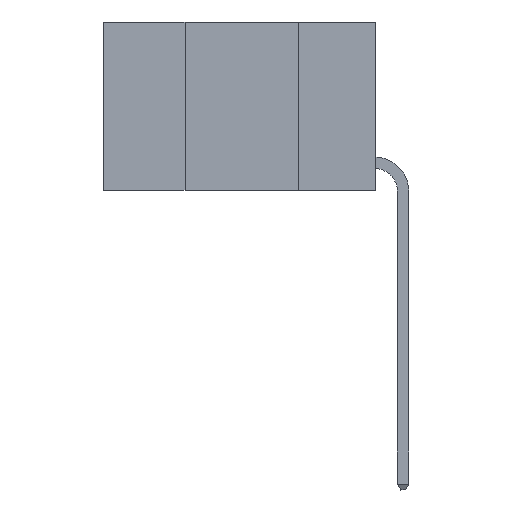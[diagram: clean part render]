
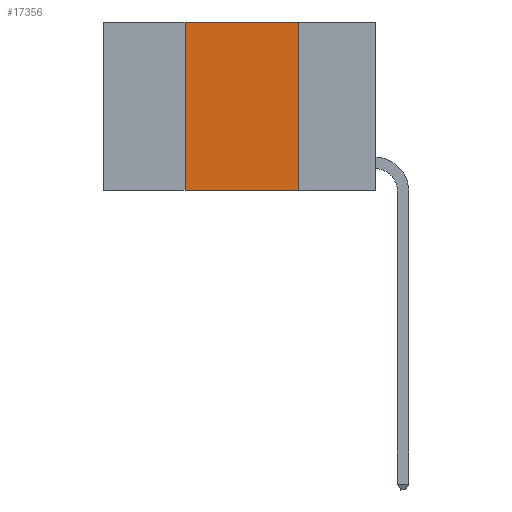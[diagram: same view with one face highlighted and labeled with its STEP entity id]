
A CAD part, left-side view. The second image highlights one B-rep face of the part: STEP entity #17356.
In plain terms, the highlighted planar face has unit normal (-1, 0, 0).
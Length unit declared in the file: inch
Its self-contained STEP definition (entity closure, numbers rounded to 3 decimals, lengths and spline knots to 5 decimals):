
#226 = EDGE_CURVE ( 'NONE', #10276, #16481, #4317, .T. ) ;
#534 = VECTOR ( 'NONE', #7224, 39.37008 ) ;
#743 = DIRECTION ( 'NONE',  ( 1., 0., 0. ) ) ;
#1006 = CARTESIAN_POINT ( 'NONE',  ( 0., 0.6, 0. ) ) ;
#1382 = CARTESIAN_POINT ( 'NONE',  ( 0., 0.42, -0.37 ) ) ;
#2932 = VECTOR ( 'NONE', #10720, 39.37008 ) ;
#3432 = CARTESIAN_POINT ( 'NONE',  ( 0., 0.42, 0. ) ) ;
#4302 = CARTESIAN_POINT ( 'NONE',  ( 0., 0.6, 0. ) ) ;
#4309 = EDGE_LOOP ( 'NONE', ( #8453, #10010, #6700, #13019 ) ) ;
#4317 = LINE ( 'NONE', #16636, #534 ) ;
#4450 = LINE ( 'NONE', #5895, #8663 ) ;
#4483 = EDGE_CURVE ( 'NONE', #10280, #13023, #10051, .T. ) ;
#4573 = CARTESIAN_POINT ( 'NONE',  ( 0., 0.17, 0. ) ) ;
#4577 = DIRECTION ( 'NONE',  ( 0., -1., 0. ) ) ;
#5895 = CARTESIAN_POINT ( 'NONE',  ( 0., 0.17, 0. ) ) ;
#6700 = ORIENTED_EDGE ( 'NONE', *, *, #14070, .F. ) ;
#6731 = EDGE_CURVE ( 'NONE', #13023, #16481, #4450, .T. ) ;
#7224 = DIRECTION ( 'NONE',  ( 0., -1., 0. ) ) ;
#8453 = ORIENTED_EDGE ( 'NONE', *, *, #6731, .F. ) ;
#8663 = VECTOR ( 'NONE', #17027, 39.37008 ) ;
#8890 = AXIS2_PLACEMENT_3D ( 'NONE', #1006, #743, #9052 ) ;
#9052 = DIRECTION ( 'NONE',  ( 0., 0., -1. ) ) ;
#9147 = FACE_OUTER_BOUND ( 'NONE', #4309, .T. ) ;
#9238 = PLANE ( 'NONE',  #8890 ) ;
#10010 = ORIENTED_EDGE ( 'NONE', *, *, #4483, .F. ) ;
#10051 = LINE ( 'NONE', #4302, #12652 ) ;
#10276 = VERTEX_POINT ( 'NONE', #1382 ) ;
#10280 = VERTEX_POINT ( 'NONE', #16709 ) ;
#10720 = DIRECTION ( 'NONE',  ( 0., 0., 1. ) ) ;
#12652 = VECTOR ( 'NONE', #4577, 39.37008 ) ;
#13019 = ORIENTED_EDGE ( 'NONE', *, *, #226, .T. ) ;
#13023 = VERTEX_POINT ( 'NONE', #4573 ) ;
#13901 = CARTESIAN_POINT ( 'NONE',  ( 0., 0.17, -0.37 ) ) ;
#14070 = EDGE_CURVE ( 'NONE', #10276, #10280, #14819, .T. ) ;
#14819 = LINE ( 'NONE', #3432, #2932 ) ;
#16481 = VERTEX_POINT ( 'NONE', #13901 ) ;
#16636 = CARTESIAN_POINT ( 'NONE',  ( 0., 0.6, -0.37 ) ) ;
#16709 = CARTESIAN_POINT ( 'NONE',  ( 0., 0.42, 0. ) ) ;
#17027 = DIRECTION ( 'NONE',  ( 0., 0., -1. ) ) ;
#17356 = ADVANCED_FACE ( 'NONE', ( #9147 ), #9238, .F. ) ;
